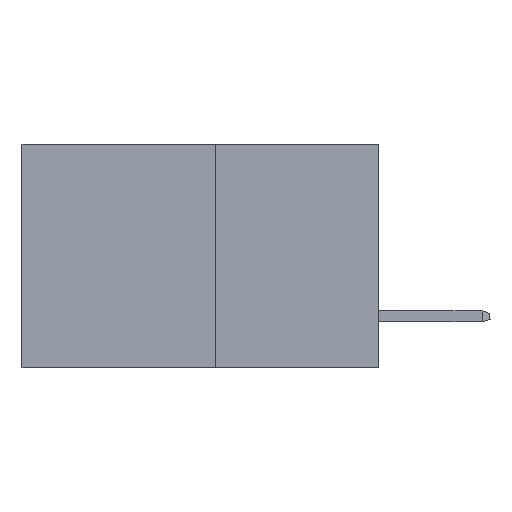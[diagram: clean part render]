
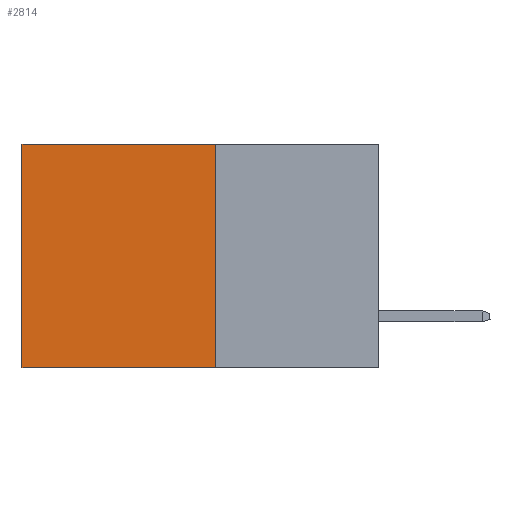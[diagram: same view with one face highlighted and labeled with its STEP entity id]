
A CAD part, left-side view. The second image highlights one B-rep face of the part: STEP entity #2814.
In plain terms, the highlighted planar face has unit normal (-1, 0, 0).
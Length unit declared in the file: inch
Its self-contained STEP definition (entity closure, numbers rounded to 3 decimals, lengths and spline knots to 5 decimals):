
#1814 = CARTESIAN_POINT ( 'NONE',  ( 0.277, 0.27, -0.37 ) ) ;
#2079 = FACE_OUTER_BOUND ( 'NONE', #21369, .T. ) ;
#2158 = DIRECTION ( 'NONE',  ( 0., 1., 0. ) ) ;
#2299 = DIRECTION ( 'NONE',  ( 0., 0., -1. ) ) ;
#2326 = AXIS2_PLACEMENT_3D ( 'NONE', #2819, #2372, #2299 ) ;
#2372 = DIRECTION ( 'NONE',  ( 1., 0., 0. ) ) ;
#2412 = PLANE ( 'NONE',  #2326 ) ;
#2814 = ADVANCED_FACE ( 'NONE', ( #2079 ), #2412, .F. ) ;
#2819 = CARTESIAN_POINT ( 'NONE',  ( 0.277, 0.27, -0.37 ) ) ;
#3065 = ORIENTED_EDGE ( 'NONE', *, *, #18904, .T. ) ;
#4053 = EDGE_CURVE ( 'NONE', #15642, #7832, #7831, .T. ) ;
#4285 = CARTESIAN_POINT ( 'NONE',  ( 0.277, 0.59, -0.37 ) ) ;
#4532 = LINE ( 'NONE', #10799, #22262 ) ;
#5566 = DIRECTION ( 'NONE',  ( 0., 1., 0. ) ) ;
#5770 = VECTOR ( 'NONE', #21621, 39.37008 ) ;
#6071 = VECTOR ( 'NONE', #6086, 39.37008 ) ;
#6086 = DIRECTION ( 'NONE',  ( 0., 0., -1. ) ) ;
#7297 = VECTOR ( 'NONE', #2158, 39.37008 ) ;
#7438 = ORIENTED_EDGE ( 'NONE', *, *, #16083, .F. ) ;
#7647 = CARTESIAN_POINT ( 'NONE',  ( 0.277, 0.27, 0. ) ) ;
#7831 = LINE ( 'NONE', #1814, #7297 ) ;
#7832 = VERTEX_POINT ( 'NONE', #20183 ) ;
#10388 = CARTESIAN_POINT ( 'NONE',  ( 0.277, 0.27, -0.37 ) ) ;
#10799 = CARTESIAN_POINT ( 'NONE',  ( 0.277, 0.27, 0. ) ) ;
#11276 = ORIENTED_EDGE ( 'NONE', *, *, #13434, .T. ) ;
#11595 = CARTESIAN_POINT ( 'NONE',  ( 0.277, 0.27, -0.37 ) ) ;
#13022 = VERTEX_POINT ( 'NONE', #21851 ) ;
#13434 = EDGE_CURVE ( 'NONE', #13022, #7832, #19765, .T. ) ;
#14648 = VERTEX_POINT ( 'NONE', #7647 ) ;
#15005 = LINE ( 'NONE', #11595, #5770 ) ;
#15642 = VERTEX_POINT ( 'NONE', #10388 ) ;
#16083 = EDGE_CURVE ( 'NONE', #14648, #15642, #15005, .T. ) ;
#18458 = ORIENTED_EDGE ( 'NONE', *, *, #4053, .F. ) ;
#18904 = EDGE_CURVE ( 'NONE', #14648, #13022, #4532, .T. ) ;
#19765 = LINE ( 'NONE', #4285, #6071 ) ;
#20183 = CARTESIAN_POINT ( 'NONE',  ( 0.277, 0.59, -0.37 ) ) ;
#21369 = EDGE_LOOP ( 'NONE', ( #11276, #18458, #7438, #3065 ) ) ;
#21621 = DIRECTION ( 'NONE',  ( 0., 0., -1. ) ) ;
#21851 = CARTESIAN_POINT ( 'NONE',  ( 0.277, 0.59, 0. ) ) ;
#22262 = VECTOR ( 'NONE', #5566, 39.37008 ) ;
